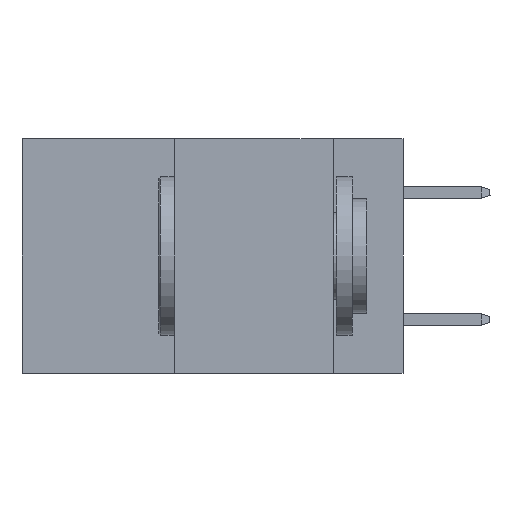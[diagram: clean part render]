
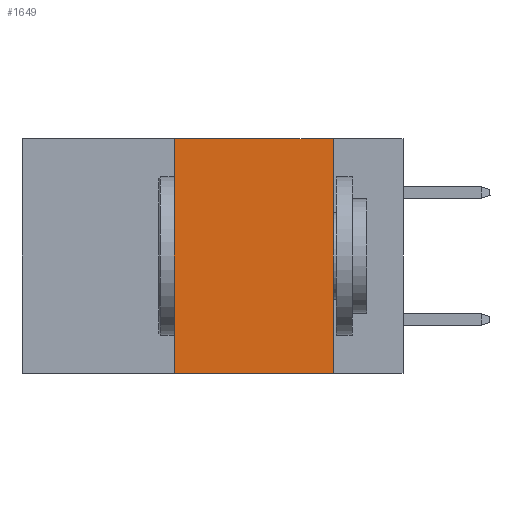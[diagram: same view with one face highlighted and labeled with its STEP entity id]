
A CAD part, left-side view. The second image highlights one B-rep face of the part: STEP entity #1649.
In plain terms, the highlighted planar face has unit normal (-1, 0, 0).
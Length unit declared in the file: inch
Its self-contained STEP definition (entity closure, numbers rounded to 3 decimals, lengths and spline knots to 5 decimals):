
#705 = FACE_OUTER_BOUND ( 'NONE', #22426, .T. ) ;
#743 = CARTESIAN_POINT ( 'NONE',  ( 0., 0.36, 0. ) ) ;
#1020 = VECTOR ( 'NONE', #7180, 39.37008 ) ;
#1649 = ADVANCED_FACE ( 'NONE', ( #705 ), #11738, .F. ) ;
#2231 = VERTEX_POINT ( 'NONE', #23236 ) ;
#2827 = LINE ( 'NONE', #8297, #7634 ) ;
#2885 = VERTEX_POINT ( 'NONE', #30747 ) ;
#4150 = ORIENTED_EDGE ( 'NONE', *, *, #20344, .T. ) ;
#6520 = DIRECTION ( 'NONE',  ( 0., 0., 1. ) ) ;
#7180 = DIRECTION ( 'NONE',  ( 0., -1., 0. ) ) ;
#7634 = VECTOR ( 'NONE', #19328, 39.37008 ) ;
#8297 = CARTESIAN_POINT ( 'NONE',  ( 0., 0.6, 0. ) ) ;
#9042 = DIRECTION ( 'NONE',  ( 1., 0., 0. ) ) ;
#9350 = CARTESIAN_POINT ( 'NONE',  ( 0., 0.11, 0. ) ) ;
#9750 = EDGE_CURVE ( 'NONE', #2231, #2885, #20317, .T. ) ;
#11738 = PLANE ( 'NONE',  #21807 ) ;
#11842 = EDGE_CURVE ( 'NONE', #17965, #33897, #20953, .T. ) ;
#12085 = DIRECTION ( 'NONE',  ( 0., 0., -1. ) ) ;
#13382 = CARTESIAN_POINT ( 'NONE',  ( 0., 0.11, -0.37 ) ) ;
#13944 = ORIENTED_EDGE ( 'NONE', *, *, #11842, .F. ) ;
#17965 = VERTEX_POINT ( 'NONE', #34070 ) ;
#18057 = VECTOR ( 'NONE', #20416, 39.37008 ) ;
#19197 = VECTOR ( 'NONE', #6520, 39.37008 ) ;
#19328 = DIRECTION ( 'NONE',  ( 0., -1., 0. ) ) ;
#20317 = LINE ( 'NONE', #743, #19197 ) ;
#20344 = EDGE_CURVE ( 'NONE', #2231, #33897, #21333, .T. ) ;
#20416 = DIRECTION ( 'NONE',  ( 0., 0., -1. ) ) ;
#20953 = LINE ( 'NONE', #9350, #18057 ) ;
#21333 = LINE ( 'NONE', #32037, #1020 ) ;
#21807 = AXIS2_PLACEMENT_3D ( 'NONE', #22829, #9042, #12085 ) ;
#22426 = EDGE_LOOP ( 'NONE', ( #13944, #34792, #34820, #4150 ) ) ;
#22829 = CARTESIAN_POINT ( 'NONE',  ( 0., 0.6, 0. ) ) ;
#23236 = CARTESIAN_POINT ( 'NONE',  ( 0., 0.36, -0.37 ) ) ;
#30747 = CARTESIAN_POINT ( 'NONE',  ( 0., 0.36, 0. ) ) ;
#32037 = CARTESIAN_POINT ( 'NONE',  ( 0., 0.6, -0.37 ) ) ;
#33897 = VERTEX_POINT ( 'NONE', #13382 ) ;
#34070 = CARTESIAN_POINT ( 'NONE',  ( 0., 0.11, 0. ) ) ;
#34372 = EDGE_CURVE ( 'NONE', #2885, #17965, #2827, .T. ) ;
#34792 = ORIENTED_EDGE ( 'NONE', *, *, #34372, .F. ) ;
#34820 = ORIENTED_EDGE ( 'NONE', *, *, #9750, .F. ) ;
